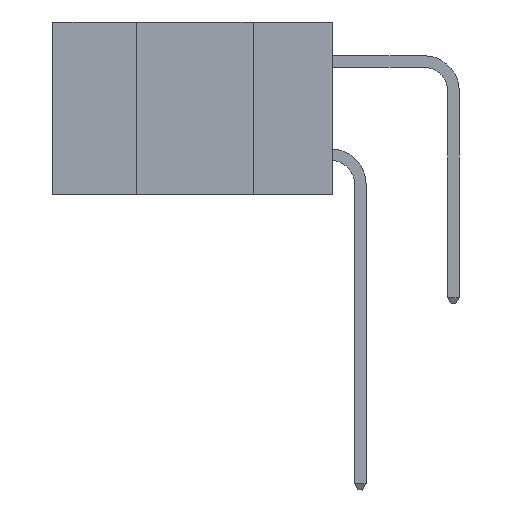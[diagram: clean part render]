
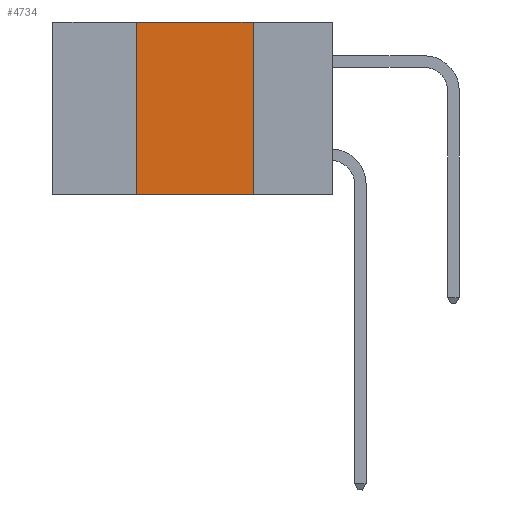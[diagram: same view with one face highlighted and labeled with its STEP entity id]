
A CAD part, left-side view. The second image highlights one B-rep face of the part: STEP entity #4734.
In plain terms, the highlighted planar face has unit normal (-1, 0, 0).
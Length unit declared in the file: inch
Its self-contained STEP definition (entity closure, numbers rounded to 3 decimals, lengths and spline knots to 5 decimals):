
#1044 = EDGE_CURVE ( 'NONE', #19041, #22401, #14848, .T. ) ;
#1387 = DIRECTION ( 'NONE',  ( 0., -1., 0. ) ) ;
#2079 = DIRECTION ( 'NONE',  ( 0., 0., 1. ) ) ;
#2333 = LINE ( 'NONE', #12015, #6522 ) ;
#3211 = VERTEX_POINT ( 'NONE', #17054 ) ;
#3616 = CARTESIAN_POINT ( 'NONE',  ( 0., 0.17, 0. ) ) ;
#4178 = CARTESIAN_POINT ( 'NONE',  ( 0., 0.17, 0. ) ) ;
#4453 = AXIS2_PLACEMENT_3D ( 'NONE', #10332, #10411, #22574 ) ;
#4734 = ADVANCED_FACE ( 'NONE', ( #21922 ), #8663, .F. ) ;
#4956 = CARTESIAN_POINT ( 'NONE',  ( 0., 0.42, 0. ) ) ;
#5859 = VECTOR ( 'NONE', #1387, 39.37008 ) ;
#6522 = VECTOR ( 'NONE', #8584, 39.37008 ) ;
#8478 = VECTOR ( 'NONE', #2079, 39.37008 ) ;
#8496 = EDGE_CURVE ( 'NONE', #18892, #19041, #2333, .T. ) ;
#8584 = DIRECTION ( 'NONE',  ( 0., -1., 0. ) ) ;
#8663 = PLANE ( 'NONE',  #4453 ) ;
#10023 = ORIENTED_EDGE ( 'NONE', *, *, #1044, .F. ) ;
#10122 = VECTOR ( 'NONE', #20463, 39.37008 ) ;
#10332 = CARTESIAN_POINT ( 'NONE',  ( 0., 0.6, 0. ) ) ;
#10411 = DIRECTION ( 'NONE',  ( 1., 0., 0. ) ) ;
#10843 = CARTESIAN_POINT ( 'NONE',  ( 0., 0.42, 0. ) ) ;
#12015 = CARTESIAN_POINT ( 'NONE',  ( 0., 0.6, 0. ) ) ;
#14742 = ORIENTED_EDGE ( 'NONE', *, *, #8496, .F. ) ;
#14848 = LINE ( 'NONE', #4178, #10122 ) ;
#16627 = LINE ( 'NONE', #10843, #8478 ) ;
#17054 = CARTESIAN_POINT ( 'NONE',  ( 0., 0.42, -0.37 ) ) ;
#17235 = ORIENTED_EDGE ( 'NONE', *, *, #20363, .T. ) ;
#18892 = VERTEX_POINT ( 'NONE', #4956 ) ;
#18949 = CARTESIAN_POINT ( 'NONE',  ( 0., 0.6, -0.37 ) ) ;
#19041 = VERTEX_POINT ( 'NONE', #3616 ) ;
#19792 = LINE ( 'NONE', #18949, #5859 ) ;
#20363 = EDGE_CURVE ( 'NONE', #3211, #22401, #19792, .T. ) ;
#20463 = DIRECTION ( 'NONE',  ( 0., 0., -1. ) ) ;
#20724 = ORIENTED_EDGE ( 'NONE', *, *, #22615, .F. ) ;
#21128 = EDGE_LOOP ( 'NONE', ( #10023, #14742, #20724, #17235 ) ) ;
#21922 = FACE_OUTER_BOUND ( 'NONE', #21128, .T. ) ;
#22399 = CARTESIAN_POINT ( 'NONE',  ( 0., 0.17, -0.37 ) ) ;
#22401 = VERTEX_POINT ( 'NONE', #22399 ) ;
#22574 = DIRECTION ( 'NONE',  ( 0., 0., -1. ) ) ;
#22615 = EDGE_CURVE ( 'NONE', #3211, #18892, #16627, .T. ) ;
